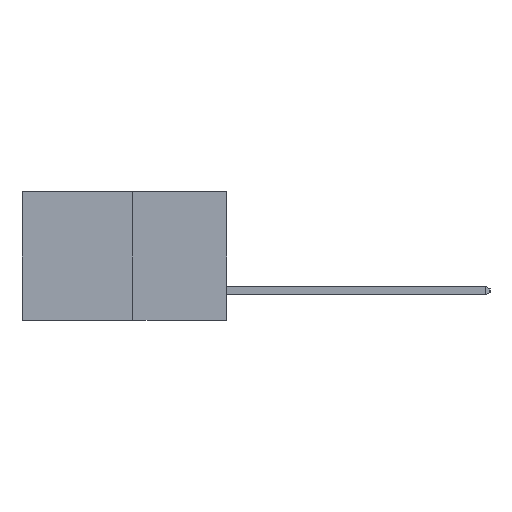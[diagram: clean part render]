
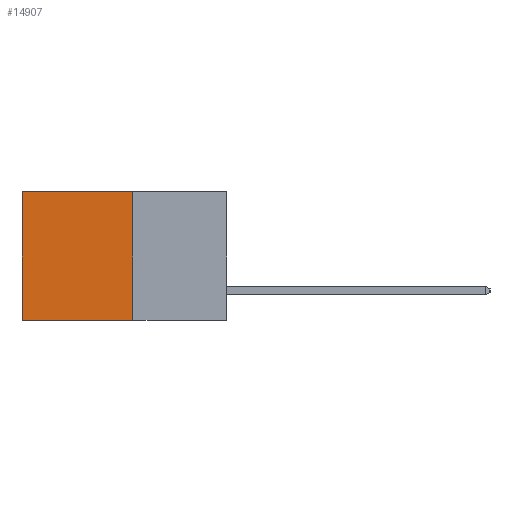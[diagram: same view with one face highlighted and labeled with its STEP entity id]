
A CAD part, left-side view. The second image highlights one B-rep face of the part: STEP entity #14907.
In plain terms, the highlighted planar face has unit normal (-1, 0, 0).
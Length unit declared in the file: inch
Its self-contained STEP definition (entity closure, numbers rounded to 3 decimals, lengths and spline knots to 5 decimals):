
#144 = DIRECTION ( 'NONE',  ( 0., 1., 0. ) ) ;
#1561 = ORIENTED_EDGE ( 'NONE', *, *, #21391, .T. ) ;
#2284 = PLANE ( 'NONE',  #21843 ) ;
#2420 = DIRECTION ( 'NONE',  ( 0., 0., -1. ) ) ;
#2579 = VECTOR ( 'NONE', #144, 39.37008 ) ;
#2601 = EDGE_CURVE ( 'NONE', #9845, #18029, #9380, .T. ) ;
#3432 = VECTOR ( 'NONE', #19016, 39.37008 ) ;
#4252 = CARTESIAN_POINT ( 'NONE',  ( 0.277, 0.27, 0. ) ) ;
#4459 = CARTESIAN_POINT ( 'NONE',  ( 0.277, 0.59, 0. ) ) ;
#5346 = LINE ( 'NONE', #5966, #18957 ) ;
#5910 = CARTESIAN_POINT ( 'NONE',  ( 0.277, 0.27, -0.37 ) ) ;
#5966 = CARTESIAN_POINT ( 'NONE',  ( 0.277, 0.59, -0.37 ) ) ;
#6536 = CARTESIAN_POINT ( 'NONE',  ( 0.277, 0.27, -0.37 ) ) ;
#6602 = CARTESIAN_POINT ( 'NONE',  ( 0.277, 0.27, -0.37 ) ) ;
#6668 = CARTESIAN_POINT ( 'NONE',  ( 0.277, 0.59, -0.37 ) ) ;
#7685 = DIRECTION ( 'NONE',  ( 0., 0., -1. ) ) ;
#8513 = DIRECTION ( 'NONE',  ( 0., 1., 0. ) ) ;
#8589 = CARTESIAN_POINT ( 'NONE',  ( 0.277, 0.27, -0.37 ) ) ;
#8800 = VECTOR ( 'NONE', #8513, 39.37008 ) ;
#9380 = LINE ( 'NONE', #8589, #8800 ) ;
#9845 = VERTEX_POINT ( 'NONE', #6536 ) ;
#9988 = ORIENTED_EDGE ( 'NONE', *, *, #12332, .F. ) ;
#10869 = CARTESIAN_POINT ( 'NONE',  ( 0.277, 0.27, 0. ) ) ;
#12332 = EDGE_CURVE ( 'NONE', #16076, #9845, #17043, .T. ) ;
#12561 = EDGE_CURVE ( 'NONE', #16076, #19167, #16186, .T. ) ;
#13099 = EDGE_LOOP ( 'NONE', ( #1561, #21470, #9988, #13398 ) ) ;
#13398 = ORIENTED_EDGE ( 'NONE', *, *, #12561, .T. ) ;
#14907 = ADVANCED_FACE ( 'NONE', ( #19233 ), #2284, .F. ) ;
#16076 = VERTEX_POINT ( 'NONE', #4252 ) ;
#16186 = LINE ( 'NONE', #10869, #2579 ) ;
#17043 = LINE ( 'NONE', #6602, #3432 ) ;
#18029 = VERTEX_POINT ( 'NONE', #6668 ) ;
#18347 = DIRECTION ( 'NONE',  ( 1., 0., 0. ) ) ;
#18957 = VECTOR ( 'NONE', #2420, 39.37008 ) ;
#19016 = DIRECTION ( 'NONE',  ( 0., 0., -1. ) ) ;
#19167 = VERTEX_POINT ( 'NONE', #4459 ) ;
#19233 = FACE_OUTER_BOUND ( 'NONE', #13099, .T. ) ;
#21391 = EDGE_CURVE ( 'NONE', #19167, #18029, #5346, .T. ) ;
#21470 = ORIENTED_EDGE ( 'NONE', *, *, #2601, .F. ) ;
#21843 = AXIS2_PLACEMENT_3D ( 'NONE', #5910, #18347, #7685 ) ;
